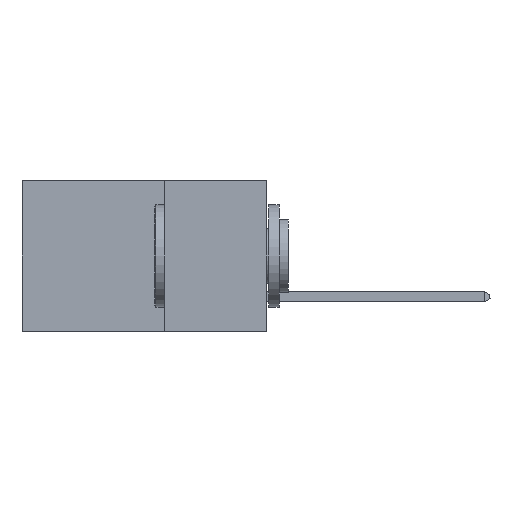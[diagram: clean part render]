
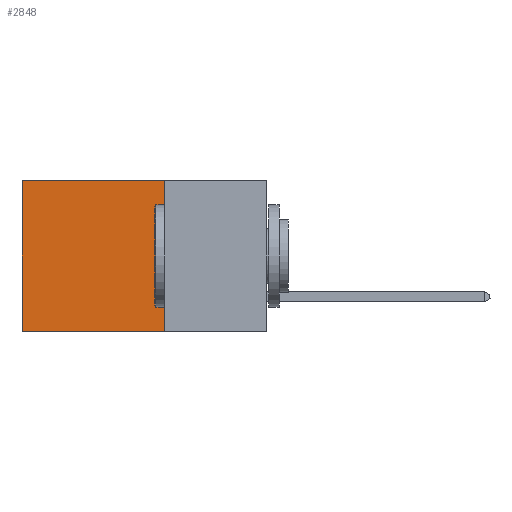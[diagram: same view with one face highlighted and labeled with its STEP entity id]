
A CAD part, left-side view. The second image highlights one B-rep face of the part: STEP entity #2848.
In plain terms, the highlighted planar face has unit normal (-1, 0, 0).
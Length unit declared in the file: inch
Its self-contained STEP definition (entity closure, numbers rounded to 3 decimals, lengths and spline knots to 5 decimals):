
#282 = PLANE ( 'NONE',  #8532 ) ;
#386 = VERTEX_POINT ( 'NONE', #31950 ) ;
#629 = LINE ( 'NONE', #10471, #17318 ) ;
#2848 = ADVANCED_FACE ( 'NONE', ( #12460 ), #282, .F. ) ;
#4027 = EDGE_CURVE ( 'NONE', #26697, #11450, #20950, .T. ) ;
#5298 = CARTESIAN_POINT ( 'NONE',  ( 0.2875, 0.25, 0. ) ) ;
#7055 = DIRECTION ( 'NONE',  ( 0., 0., -1. ) ) ;
#7430 = VERTEX_POINT ( 'NONE', #17039 ) ;
#8532 = AXIS2_PLACEMENT_3D ( 'NONE', #5298, #22670, #25276 ) ;
#9450 = LINE ( 'NONE', #17801, #26571 ) ;
#9513 = ORIENTED_EDGE ( 'NONE', *, *, #24928, .T. ) ;
#10320 = ORIENTED_EDGE ( 'NONE', *, *, #18615, .F. ) ;
#10471 = CARTESIAN_POINT ( 'NONE',  ( 0.2875, 0.25, -0.37 ) ) ;
#11450 = VERTEX_POINT ( 'NONE', #20667 ) ;
#12460 = FACE_OUTER_BOUND ( 'NONE', #21380, .T. ) ;
#13242 = LINE ( 'NONE', #19424, #15574 ) ;
#15020 = EDGE_CURVE ( 'NONE', #386, #7430, #13242, .T. ) ;
#15574 = VECTOR ( 'NONE', #7055, 39.37008 ) ;
#16557 = ORIENTED_EDGE ( 'NONE', *, *, #4027, .T. ) ;
#17039 = CARTESIAN_POINT ( 'NONE',  ( 0.2875, 0.25, -0.37 ) ) ;
#17318 = VECTOR ( 'NONE', #25141, 39.37008 ) ;
#17589 = CARTESIAN_POINT ( 'NONE',  ( 0.2875, 0.6, 0. ) ) ;
#17801 = CARTESIAN_POINT ( 'NONE',  ( 0.2875, 0.25, 0. ) ) ;
#18615 = EDGE_CURVE ( 'NONE', #7430, #11450, #629, .T. ) ;
#19424 = CARTESIAN_POINT ( 'NONE',  ( 0.2875, 0.25, 0. ) ) ;
#20667 = CARTESIAN_POINT ( 'NONE',  ( 0.2875, 0.6, -0.37 ) ) ;
#20764 = DIRECTION ( 'NONE',  ( 0., 0., -1. ) ) ;
#20950 = LINE ( 'NONE', #20970, #24465 ) ;
#20970 = CARTESIAN_POINT ( 'NONE',  ( 0.2875, 0.6, 0. ) ) ;
#21380 = EDGE_LOOP ( 'NONE', ( #16557, #10320, #25043, #9513 ) ) ;
#22670 = DIRECTION ( 'NONE',  ( 1., 0., 0. ) ) ;
#24465 = VECTOR ( 'NONE', #20764, 39.37008 ) ;
#24928 = EDGE_CURVE ( 'NONE', #386, #26697, #9450, .T. ) ;
#25009 = DIRECTION ( 'NONE',  ( 0., 1., 0. ) ) ;
#25043 = ORIENTED_EDGE ( 'NONE', *, *, #15020, .F. ) ;
#25141 = DIRECTION ( 'NONE',  ( 0., 1., 0. ) ) ;
#25276 = DIRECTION ( 'NONE',  ( 0., 0., -1. ) ) ;
#26571 = VECTOR ( 'NONE', #25009, 39.37008 ) ;
#26697 = VERTEX_POINT ( 'NONE', #17589 ) ;
#31950 = CARTESIAN_POINT ( 'NONE',  ( 0.2875, 0.25, 0. ) ) ;
